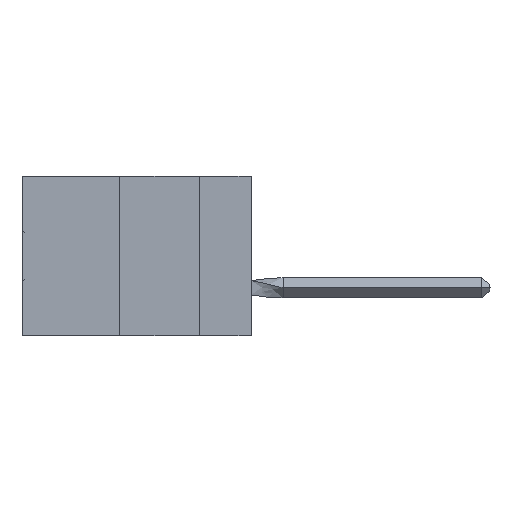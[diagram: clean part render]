
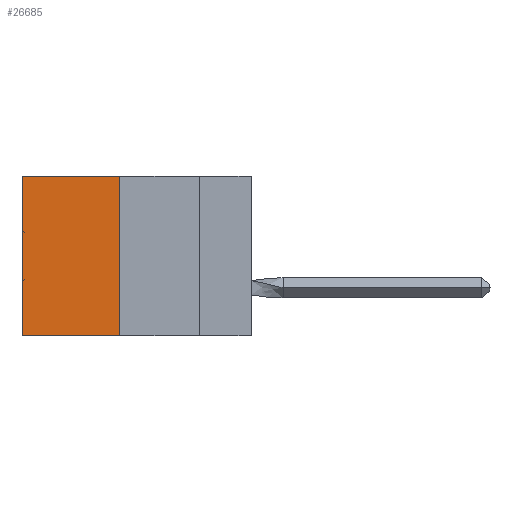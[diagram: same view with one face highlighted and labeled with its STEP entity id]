
A CAD part, left-side view. The second image highlights one B-rep face of the part: STEP entity #26685.
In plain terms, the highlighted planar face has unit normal (-1, 0, 0).
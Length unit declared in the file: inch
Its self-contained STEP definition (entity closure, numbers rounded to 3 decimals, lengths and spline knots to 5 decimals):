
#742 = LINE ( 'NONE', #39407, #12967 ) ;
#1780 = FACE_OUTER_BOUND ( 'NONE', #39035, .T. ) ;
#5847 = EDGE_CURVE ( 'NONE', #21426, #46771, #742, .T. ) ;
#6558 = DIRECTION ( 'NONE',  ( 1., 0., 0. ) ) ;
#10172 = DIRECTION ( 'NONE',  ( 0., 0., -1. ) ) ;
#12774 = DIRECTION ( 'NONE',  ( 0., 0., -1. ) ) ;
#12967 = VECTOR ( 'NONE', #15129, 39.37008 ) ;
#15102 = VECTOR ( 'NONE', #12774, 39.37008 ) ;
#15129 = DIRECTION ( 'NONE',  ( 0., 1., 0. ) ) ;
#17668 = ORIENTED_EDGE ( 'NONE', *, *, #52438, .T. ) ;
#17724 = CARTESIAN_POINT ( 'NONE',  ( 0.305, 0.72, -0.5 ) ) ;
#20858 = CARTESIAN_POINT ( 'NONE',  ( 0.305, 0.413, -0.5 ) ) ;
#21330 = ORIENTED_EDGE ( 'NONE', *, *, #25563, .F. ) ;
#21426 = VERTEX_POINT ( 'NONE', #38797 ) ;
#25563 = EDGE_CURVE ( 'NONE', #21426, #35361, #26036, .T. ) ;
#25652 = VECTOR ( 'NONE', #43352, 39.37008 ) ;
#26036 = LINE ( 'NONE', #20858, #15102 ) ;
#26685 = ADVANCED_FACE ( 'NONE', ( #1780 ), #31361, .F. ) ;
#31361 = PLANE ( 'NONE',  #38709 ) ;
#31467 = VECTOR ( 'NONE', #10172, 39.37008 ) ;
#31470 = CARTESIAN_POINT ( 'NONE',  ( 0.305, 0.413, -0.5 ) ) ;
#32787 = VERTEX_POINT ( 'NONE', #33020 ) ;
#33020 = CARTESIAN_POINT ( 'NONE',  ( 0.305, 0.72, -0.5 ) ) ;
#33255 = EDGE_CURVE ( 'NONE', #35361, #32787, #50061, .T. ) ;
#33850 = CARTESIAN_POINT ( 'NONE',  ( 0.305, 0.72, 0. ) ) ;
#34275 = ORIENTED_EDGE ( 'NONE', *, *, #5847, .T. ) ;
#35249 = CARTESIAN_POINT ( 'NONE',  ( 0.305, 0.413, -0.5 ) ) ;
#35361 = VERTEX_POINT ( 'NONE', #31470 ) ;
#38709 = AXIS2_PLACEMENT_3D ( 'NONE', #47520, #6558, #43576 ) ;
#38797 = CARTESIAN_POINT ( 'NONE',  ( 0.305, 0.413, 0. ) ) ;
#39035 = EDGE_LOOP ( 'NONE', ( #17668, #50952, #21330, #34275 ) ) ;
#39407 = CARTESIAN_POINT ( 'NONE',  ( 0.305, 0.413, 0. ) ) ;
#43352 = DIRECTION ( 'NONE',  ( 0., 1., 0. ) ) ;
#43576 = DIRECTION ( 'NONE',  ( 0., 0., -1. ) ) ;
#44977 = LINE ( 'NONE', #17724, #31467 ) ;
#46771 = VERTEX_POINT ( 'NONE', #33850 ) ;
#47520 = CARTESIAN_POINT ( 'NONE',  ( 0.305, 0.413, -0.5 ) ) ;
#50061 = LINE ( 'NONE', #35249, #25652 ) ;
#50952 = ORIENTED_EDGE ( 'NONE', *, *, #33255, .F. ) ;
#52438 = EDGE_CURVE ( 'NONE', #46771, #32787, #44977, .T. ) ;
